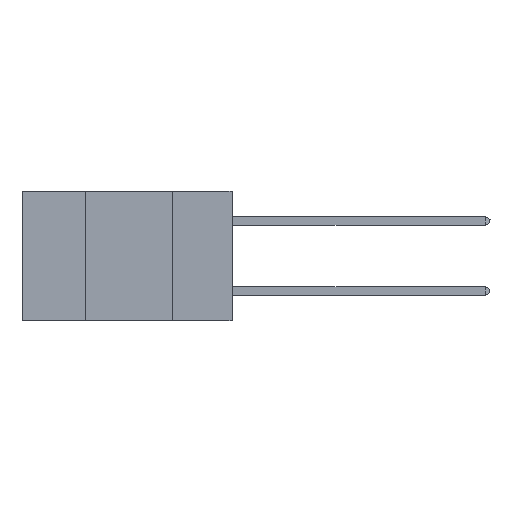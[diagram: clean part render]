
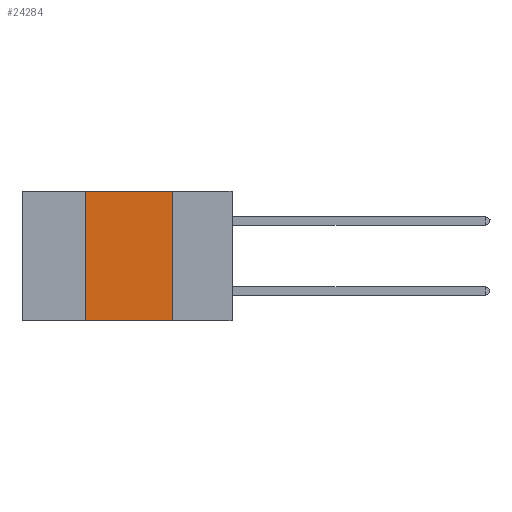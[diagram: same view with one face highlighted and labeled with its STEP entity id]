
A CAD part, left-side view. The second image highlights one B-rep face of the part: STEP entity #24284.
In plain terms, the highlighted planar face has unit normal (-1, 0, 0).
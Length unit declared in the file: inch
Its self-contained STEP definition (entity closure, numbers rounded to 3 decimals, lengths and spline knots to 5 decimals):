
#2578 = ORIENTED_EDGE ( 'NONE', *, *, #43822, .F. ) ;
#4877 = DIRECTION ( 'NONE',  ( 0., 0., -1. ) ) ;
#5434 = AXIS2_PLACEMENT_3D ( 'NONE', #12220, #16277, #4877 ) ;
#8179 = VERTEX_POINT ( 'NONE', #9053 ) ;
#9053 = CARTESIAN_POINT ( 'NONE',  ( 0., 0.42, -0.37 ) ) ;
#9943 = VECTOR ( 'NONE', #24262, 39.37008 ) ;
#10361 = DIRECTION ( 'NONE',  ( 0., 0., 1. ) ) ;
#11337 = EDGE_LOOP ( 'NONE', ( #21549, #29642, #2578, #37191 ) ) ;
#12220 = CARTESIAN_POINT ( 'NONE',  ( 0., 0.6, 0. ) ) ;
#12446 = EDGE_CURVE ( 'NONE', #22689, #32217, #12963, .T. ) ;
#12963 = LINE ( 'NONE', #42488, #20589 ) ;
#14387 = CARTESIAN_POINT ( 'NONE',  ( 0., 0.42, 0. ) ) ;
#14655 = VECTOR ( 'NONE', #32701, 39.37008 ) ;
#16277 = DIRECTION ( 'NONE',  ( 1., 0., 0. ) ) ;
#18929 = VERTEX_POINT ( 'NONE', #40568 ) ;
#19322 = CARTESIAN_POINT ( 'NONE',  ( 0., 0.17, -0.37 ) ) ;
#20589 = VECTOR ( 'NONE', #43181, 39.37008 ) ;
#21549 = ORIENTED_EDGE ( 'NONE', *, *, #12446, .F. ) ;
#22689 = VERTEX_POINT ( 'NONE', #38941 ) ;
#24262 = DIRECTION ( 'NONE',  ( 0., -1., 0. ) ) ;
#24284 = ADVANCED_FACE ( 'NONE', ( #27008 ), #30340, .F. ) ;
#26130 = EDGE_CURVE ( 'NONE', #18929, #22689, #40544, .T. ) ;
#27008 = FACE_OUTER_BOUND ( 'NONE', #11337, .T. ) ;
#27626 = LINE ( 'NONE', #34527, #9943 ) ;
#29642 = ORIENTED_EDGE ( 'NONE', *, *, #26130, .F. ) ;
#30340 = PLANE ( 'NONE',  #5434 ) ;
#31501 = VECTOR ( 'NONE', #10361, 39.37008 ) ;
#32217 = VERTEX_POINT ( 'NONE', #19322 ) ;
#32701 = DIRECTION ( 'NONE',  ( 0., -1., 0. ) ) ;
#34527 = CARTESIAN_POINT ( 'NONE',  ( 0., 0.6, -0.37 ) ) ;
#37191 = ORIENTED_EDGE ( 'NONE', *, *, #38354, .T. ) ;
#38354 = EDGE_CURVE ( 'NONE', #8179, #32217, #27626, .T. ) ;
#38941 = CARTESIAN_POINT ( 'NONE',  ( 0., 0.17, 0. ) ) ;
#39520 = LINE ( 'NONE', #14387, #31501 ) ;
#40544 = LINE ( 'NONE', #43166, #14655 ) ;
#40568 = CARTESIAN_POINT ( 'NONE',  ( 0., 0.42, 0. ) ) ;
#42488 = CARTESIAN_POINT ( 'NONE',  ( 0., 0.17, 0. ) ) ;
#43166 = CARTESIAN_POINT ( 'NONE',  ( 0., 0.6, 0. ) ) ;
#43181 = DIRECTION ( 'NONE',  ( 0., 0., -1. ) ) ;
#43822 = EDGE_CURVE ( 'NONE', #8179, #18929, #39520, .T. ) ;
